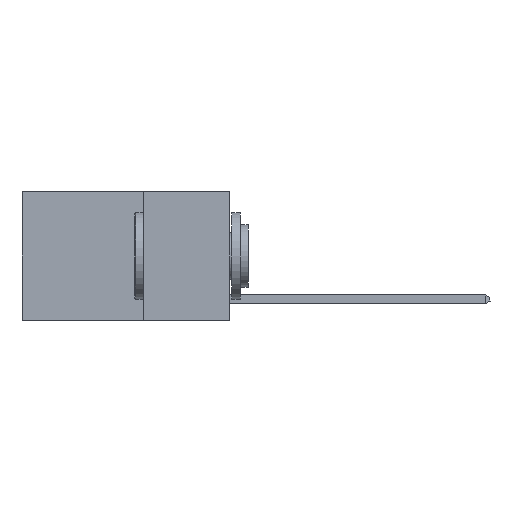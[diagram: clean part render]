
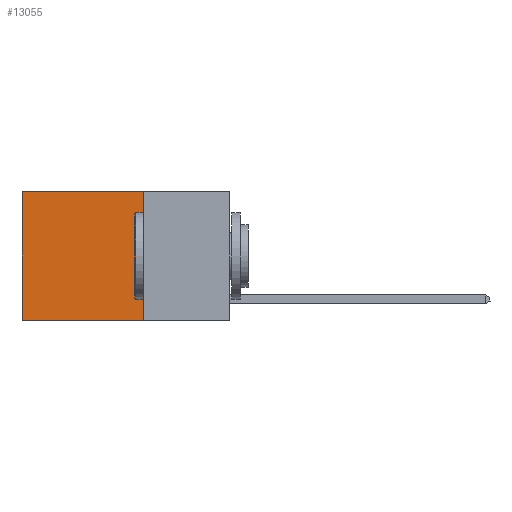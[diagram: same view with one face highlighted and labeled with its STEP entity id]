
A CAD part, left-side view. The second image highlights one B-rep face of the part: STEP entity #13055.
In plain terms, the highlighted planar face has unit normal (-1, 0, 0).
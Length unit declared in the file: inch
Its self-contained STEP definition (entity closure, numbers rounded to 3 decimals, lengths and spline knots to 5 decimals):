
#650 = VECTOR ( 'NONE', #858, 39.37008 ) ;
#858 = DIRECTION ( 'NONE',  ( 0., 0., -1. ) ) ;
#1533 = ORIENTED_EDGE ( 'NONE', *, *, #8168, .T. ) ;
#1699 = PLANE ( 'NONE',  #11432 ) ;
#1808 = LINE ( 'NONE', #13707, #7952 ) ;
#1990 = VERTEX_POINT ( 'NONE', #11517 ) ;
#2561 = DIRECTION ( 'NONE',  ( 0., 1., 0. ) ) ;
#3414 = ORIENTED_EDGE ( 'NONE', *, *, #17898, .F. ) ;
#3503 = FACE_OUTER_BOUND ( 'NONE', #8629, .T. ) ;
#4221 = DIRECTION ( 'NONE',  ( 0., 0., -1. ) ) ;
#4545 = CARTESIAN_POINT ( 'NONE',  ( 0.2625, 0.25, 0. ) ) ;
#4670 = ORIENTED_EDGE ( 'NONE', *, *, #13820, .F. ) ;
#5400 = CARTESIAN_POINT ( 'NONE',  ( 0.2625, 0.25, 0. ) ) ;
#6836 = VERTEX_POINT ( 'NONE', #9411 ) ;
#6924 = CARTESIAN_POINT ( 'NONE',  ( 0.2625, 0.25, 0. ) ) ;
#7952 = VECTOR ( 'NONE', #8072, 39.37008 ) ;
#8072 = DIRECTION ( 'NONE',  ( 0., 1., 0. ) ) ;
#8168 = EDGE_CURVE ( 'NONE', #17486, #1990, #17266, .T. ) ;
#8629 = EDGE_LOOP ( 'NONE', ( #13830, #3414, #4670, #1533 ) ) ;
#8682 = LINE ( 'NONE', #6924, #9116 ) ;
#9116 = VECTOR ( 'NONE', #4221, 39.37008 ) ;
#9411 = CARTESIAN_POINT ( 'NONE',  ( 0.2625, 0.25, -0.37 ) ) ;
#10472 = DIRECTION ( 'NONE',  ( 0., 0., -1. ) ) ;
#10536 = CARTESIAN_POINT ( 'NONE',  ( 0.2625, 0.6, 0. ) ) ;
#10549 = VECTOR ( 'NONE', #2561, 39.37008 ) ;
#10819 = EDGE_CURVE ( 'NONE', #1990, #14121, #15648, .T. ) ;
#11432 = AXIS2_PLACEMENT_3D ( 'NONE', #4545, #11759, #10472 ) ;
#11517 = CARTESIAN_POINT ( 'NONE',  ( 0.2625, 0.6, 0. ) ) ;
#11759 = DIRECTION ( 'NONE',  ( 1., 0., 0. ) ) ;
#13055 = ADVANCED_FACE ( 'NONE', ( #3503 ), #1699, .F. ) ;
#13707 = CARTESIAN_POINT ( 'NONE',  ( 0.2625, 0.25, -0.37 ) ) ;
#13820 = EDGE_CURVE ( 'NONE', #17486, #6836, #8682, .T. ) ;
#13830 = ORIENTED_EDGE ( 'NONE', *, *, #10819, .T. ) ;
#14032 = CARTESIAN_POINT ( 'NONE',  ( 0.2625, 0.25, 0. ) ) ;
#14121 = VERTEX_POINT ( 'NONE', #16242 ) ;
#15648 = LINE ( 'NONE', #10536, #650 ) ;
#16242 = CARTESIAN_POINT ( 'NONE',  ( 0.2625, 0.6, -0.37 ) ) ;
#17266 = LINE ( 'NONE', #5400, #10549 ) ;
#17486 = VERTEX_POINT ( 'NONE', #14032 ) ;
#17898 = EDGE_CURVE ( 'NONE', #6836, #14121, #1808, .T. ) ;
